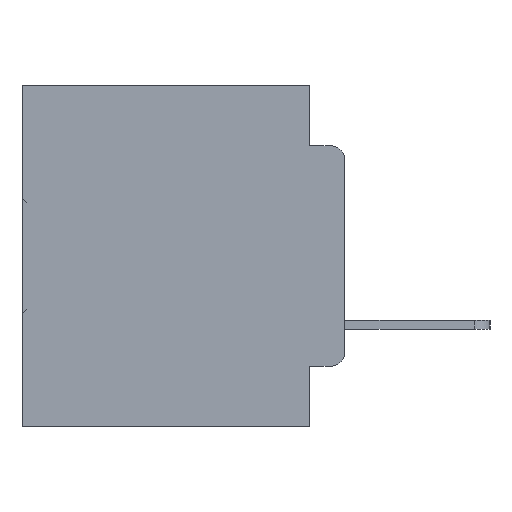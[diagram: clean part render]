
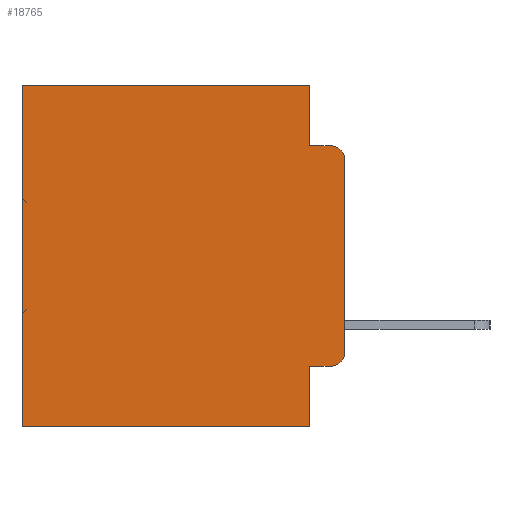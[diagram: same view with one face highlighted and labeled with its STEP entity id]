
A CAD part, left-side view. The second image highlights one B-rep face of the part: STEP entity #18765.
In plain terms, the highlighted planar face has unit normal (-1, 0, 0).
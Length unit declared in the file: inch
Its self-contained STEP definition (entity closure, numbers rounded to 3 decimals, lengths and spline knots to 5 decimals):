
#171 = CARTESIAN_POINT ( 'NONE',  ( 0.298, 0.051, 0. ) ) ;
#228 = EDGE_CURVE ( 'NONE', #1710, #2694, #25317, .T. ) ;
#439 = CARTESIAN_POINT ( 'NONE',  ( 0.298, 0.473, 0. ) ) ;
#508 = CARTESIAN_POINT ( 'NONE',  ( 0.298, 0.051, 0. ) ) ;
#640 = VECTOR ( 'NONE', #10789, 39.37008 ) ;
#1212 = CARTESIAN_POINT ( 'NONE',  ( 0.298, 0., 0. ) ) ;
#1353 = LINE ( 'NONE', #5544, #22961 ) ;
#1507 = LINE ( 'NONE', #31894, #23094 ) ;
#1710 = VERTEX_POINT ( 'NONE', #171 ) ;
#2111 = DIRECTION ( 'NONE',  ( 0., 0., -1. ) ) ;
#2170 = EDGE_CURVE ( 'NONE', #2694, #21934, #20123, .T. ) ;
#2182 = DIRECTION ( 'NONE',  ( 0., 0., -1. ) ) ;
#2332 = DIRECTION ( 'NONE',  ( 0., -1., 0. ) ) ;
#2694 = VERTEX_POINT ( 'NONE', #26878 ) ;
#3816 = VERTEX_POINT ( 'NONE', #20240 ) ;
#5522 = LINE ( 'NONE', #24760, #26768 ) ;
#5544 = CARTESIAN_POINT ( 'NONE',  ( 0.298, 0.051, 0. ) ) ;
#5607 = LINE ( 'NONE', #508, #26841 ) ;
#6153 = VECTOR ( 'NONE', #9944, 39.37008 ) ;
#6379 = CARTESIAN_POINT ( 'NONE',  ( 0.298, 0.051, -0.4115 ) ) ;
#6484 = VERTEX_POINT ( 'NONE', #10766 ) ;
#6833 = EDGE_CURVE ( 'NONE', #3816, #6484, #13816, .T. ) ;
#7314 = CARTESIAN_POINT ( 'NONE',  ( 0.298, 0.02, -0.0885 ) ) ;
#7675 = ORIENTED_EDGE ( 'NONE', *, *, #35108, .F. ) ;
#7726 = CARTESIAN_POINT ( 'NONE',  ( 0.298, 0., 0. ) ) ;
#8560 = CIRCLE ( 'NONE', #17949, 0.02 ) ;
#8609 = VERTEX_POINT ( 'NONE', #7314 ) ;
#9345 = LINE ( 'NONE', #7726, #640 ) ;
#9944 = DIRECTION ( 'NONE',  ( 0., -1., 0. ) ) ;
#10305 = VERTEX_POINT ( 'NONE', #25029 ) ;
#10341 = VERTEX_POINT ( 'NONE', #23234 ) ;
#10548 = CIRCLE ( 'NONE', #23548, 0.02 ) ;
#10766 = CARTESIAN_POINT ( 'NONE',  ( 0.298, 0.02, -0.4115 ) ) ;
#10779 = EDGE_CURVE ( 'NONE', #10305, #21934, #1507, .T. ) ;
#10789 = DIRECTION ( 'NONE',  ( 0., 0., -1. ) ) ;
#12524 = CARTESIAN_POINT ( 'NONE',  ( 0.298, 0.02, -0.3915 ) ) ;
#12802 = VECTOR ( 'NONE', #19319, 39.37008 ) ;
#13482 = ORIENTED_EDGE ( 'NONE', *, *, #228, .T. ) ;
#13816 = LINE ( 'NONE', #6379, #6153 ) ;
#14556 = DIRECTION ( 'NONE',  ( 0., 1., 0. ) ) ;
#14878 = VERTEX_POINT ( 'NONE', #18931 ) ;
#14948 = EDGE_CURVE ( 'NONE', #14878, #8609, #8560, .T. ) ;
#15304 = DIRECTION ( 'NONE',  ( 0., 0., -1. ) ) ;
#16133 = EDGE_CURVE ( 'NONE', #14878, #10341, #9345, .T. ) ;
#16428 = PLANE ( 'NONE',  #24743 ) ;
#17176 = ORIENTED_EDGE ( 'NONE', *, *, #14948, .T. ) ;
#17949 = AXIS2_PLACEMENT_3D ( 'NONE', #34910, #19253, #2182 ) ;
#18231 = VECTOR ( 'NONE', #14556, 39.37008 ) ;
#18765 = ADVANCED_FACE ( 'NONE', ( #24446 ), #16428, .F. ) ;
#18931 = CARTESIAN_POINT ( 'NONE',  ( 0.298, 0., -0.1085 ) ) ;
#19189 = DIRECTION ( 'NONE',  ( 1., 0., 0. ) ) ;
#19253 = DIRECTION ( 'NONE',  ( -1., 0., 0. ) ) ;
#19319 = DIRECTION ( 'NONE',  ( 0., 0., -1. ) ) ;
#20123 = LINE ( 'NONE', #439, #12802 ) ;
#20240 = CARTESIAN_POINT ( 'NONE',  ( 0.298, 0.051, -0.4115 ) ) ;
#21155 = EDGE_CURVE ( 'NONE', #1710, #23293, #1353, .T. ) ;
#21934 = VERTEX_POINT ( 'NONE', #28291 ) ;
#22961 = VECTOR ( 'NONE', #24982, 39.37008 ) ;
#22975 = EDGE_LOOP ( 'NONE', ( #24722, #17176, #7675, #32923, #13482, #26204, #34624, #28251, #32312, #27426 ) ) ;
#23094 = VECTOR ( 'NONE', #31860, 39.37008 ) ;
#23234 = CARTESIAN_POINT ( 'NONE',  ( 0.298, 0., -0.3915 ) ) ;
#23293 = VERTEX_POINT ( 'NONE', #31064 ) ;
#23548 = AXIS2_PLACEMENT_3D ( 'NONE', #12524, #31306, #15304 ) ;
#24446 = FACE_OUTER_BOUND ( 'NONE', #22975, .T. ) ;
#24722 = ORIENTED_EDGE ( 'NONE', *, *, #16133, .F. ) ;
#24743 = AXIS2_PLACEMENT_3D ( 'NONE', #29601, #19189, #2111 ) ;
#24760 = CARTESIAN_POINT ( 'NONE',  ( 0.298, 0.051, -0.0885 ) ) ;
#24982 = DIRECTION ( 'NONE',  ( 0., 0., -1. ) ) ;
#25029 = CARTESIAN_POINT ( 'NONE',  ( 0.298, 0.051, -0.5 ) ) ;
#25317 = LINE ( 'NONE', #1212, #18231 ) ;
#26204 = ORIENTED_EDGE ( 'NONE', *, *, #2170, .T. ) ;
#26768 = VECTOR ( 'NONE', #2332, 39.37008 ) ;
#26841 = VECTOR ( 'NONE', #30979, 39.37008 ) ;
#26878 = CARTESIAN_POINT ( 'NONE',  ( 0.298, 0.473, 0. ) ) ;
#27426 = ORIENTED_EDGE ( 'NONE', *, *, #34685, .T. ) ;
#28251 = ORIENTED_EDGE ( 'NONE', *, *, #32360, .F. ) ;
#28291 = CARTESIAN_POINT ( 'NONE',  ( 0.298, 0.473, -0.5 ) ) ;
#29601 = CARTESIAN_POINT ( 'NONE',  ( 0.298, 0., 0. ) ) ;
#30979 = DIRECTION ( 'NONE',  ( 0., 0., -1. ) ) ;
#31064 = CARTESIAN_POINT ( 'NONE',  ( 0.298, 0.051, -0.0885 ) ) ;
#31306 = DIRECTION ( 'NONE',  ( -1., 0., 0. ) ) ;
#31860 = DIRECTION ( 'NONE',  ( 0., 1., 0. ) ) ;
#31894 = CARTESIAN_POINT ( 'NONE',  ( 0.298, 0., -0.5 ) ) ;
#32312 = ORIENTED_EDGE ( 'NONE', *, *, #6833, .T. ) ;
#32360 = EDGE_CURVE ( 'NONE', #3816, #10305, #5607, .T. ) ;
#32923 = ORIENTED_EDGE ( 'NONE', *, *, #21155, .F. ) ;
#34624 = ORIENTED_EDGE ( 'NONE', *, *, #10779, .F. ) ;
#34685 = EDGE_CURVE ( 'NONE', #6484, #10341, #10548, .T. ) ;
#34910 = CARTESIAN_POINT ( 'NONE',  ( 0.298, 0.02, -0.1085 ) ) ;
#35108 = EDGE_CURVE ( 'NONE', #23293, #8609, #5522, .T. ) ;
